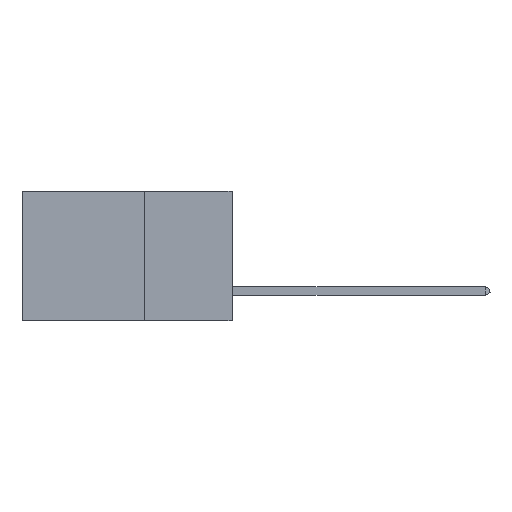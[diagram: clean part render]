
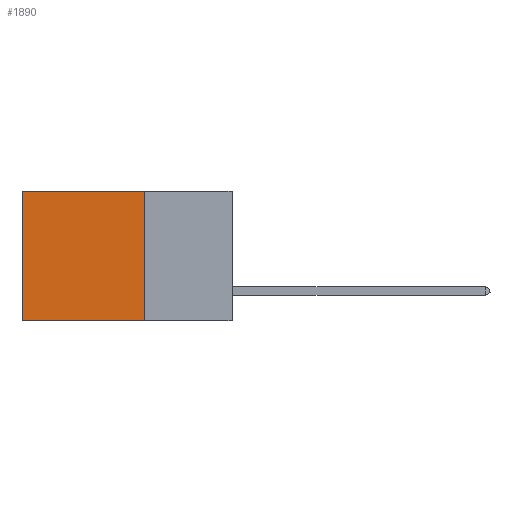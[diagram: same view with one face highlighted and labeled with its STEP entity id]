
A CAD part, left-side view. The second image highlights one B-rep face of the part: STEP entity #1890.
In plain terms, the highlighted planar face has unit normal (-1, 0, 0).
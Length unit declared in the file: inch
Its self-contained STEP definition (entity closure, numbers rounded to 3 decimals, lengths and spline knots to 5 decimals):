
#1890 = ADVANCED_FACE ( 'NONE', ( #31570 ), #35648, .F. ) ;
#2152 = LINE ( 'NONE', #38555, #36107 ) ;
#5045 = VERTEX_POINT ( 'NONE', #18680 ) ;
#5889 = VECTOR ( 'NONE', #38910, 39.37008 ) ;
#9167 = VECTOR ( 'NONE', #15544, 39.37008 ) ;
#9844 = VERTEX_POINT ( 'NONE', #15205 ) ;
#9910 = ORIENTED_EDGE ( 'NONE', *, *, #22827, .F. ) ;
#11831 = CARTESIAN_POINT ( 'NONE',  ( 0.2875, 0.25, -0.37 ) ) ;
#15205 = CARTESIAN_POINT ( 'NONE',  ( 0.2875, 0.6, -0.37 ) ) ;
#15544 = DIRECTION ( 'NONE',  ( 0., 1., 0. ) ) ;
#16704 = EDGE_LOOP ( 'NONE', ( #33248, #19544, #9910, #31236 ) ) ;
#17170 = DIRECTION ( 'NONE',  ( 1., 0., 0. ) ) ;
#17501 = EDGE_CURVE ( 'NONE', #36285, #36957, #17547, .T. ) ;
#17547 = LINE ( 'NONE', #34492, #9167 ) ;
#18680 = CARTESIAN_POINT ( 'NONE',  ( 0.2875, 0.25, -0.37 ) ) ;
#19349 = VECTOR ( 'NONE', #40567, 39.37008 ) ;
#19544 = ORIENTED_EDGE ( 'NONE', *, *, #29308, .F. ) ;
#19962 = CARTESIAN_POINT ( 'NONE',  ( 0.2875, 0.25, 0. ) ) ;
#22675 = LINE ( 'NONE', #38634, #5889 ) ;
#22827 = EDGE_CURVE ( 'NONE', #36285, #5045, #2152, .T. ) ;
#22872 = DIRECTION ( 'NONE',  ( 0., 0., -1. ) ) ;
#23730 = CARTESIAN_POINT ( 'NONE',  ( 0.2875, 0.6, 0. ) ) ;
#23826 = DIRECTION ( 'NONE',  ( 0., 0., -1. ) ) ;
#24188 = CARTESIAN_POINT ( 'NONE',  ( 0.2875, 0.25, 0. ) ) ;
#25490 = EDGE_CURVE ( 'NONE', #36957, #9844, #22675, .T. ) ;
#29239 = LINE ( 'NONE', #11831, #19349 ) ;
#29308 = EDGE_CURVE ( 'NONE', #5045, #9844, #29239, .T. ) ;
#31236 = ORIENTED_EDGE ( 'NONE', *, *, #17501, .T. ) ;
#31570 = FACE_OUTER_BOUND ( 'NONE', #16704, .T. ) ;
#33248 = ORIENTED_EDGE ( 'NONE', *, *, #25490, .T. ) ;
#34492 = CARTESIAN_POINT ( 'NONE',  ( 0.2875, 0.25, 0. ) ) ;
#35648 = PLANE ( 'NONE',  #38537 ) ;
#36107 = VECTOR ( 'NONE', #22872, 39.37008 ) ;
#36285 = VERTEX_POINT ( 'NONE', #24188 ) ;
#36957 = VERTEX_POINT ( 'NONE', #23730 ) ;
#38537 = AXIS2_PLACEMENT_3D ( 'NONE', #19962, #17170, #23826 ) ;
#38555 = CARTESIAN_POINT ( 'NONE',  ( 0.2875, 0.25, 0. ) ) ;
#38634 = CARTESIAN_POINT ( 'NONE',  ( 0.2875, 0.6, 0. ) ) ;
#38910 = DIRECTION ( 'NONE',  ( 0., 0., -1. ) ) ;
#40567 = DIRECTION ( 'NONE',  ( 0., 1., 0. ) ) ;
